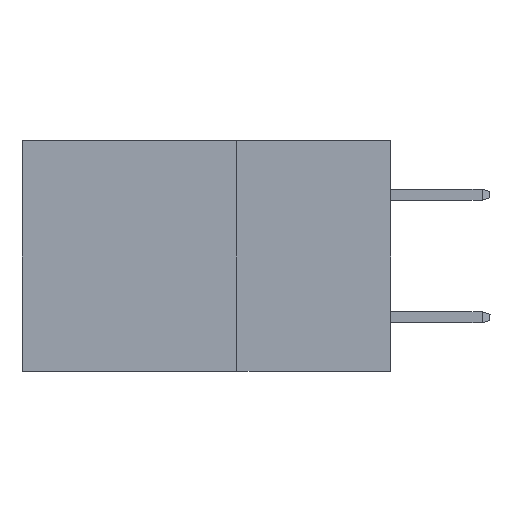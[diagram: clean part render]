
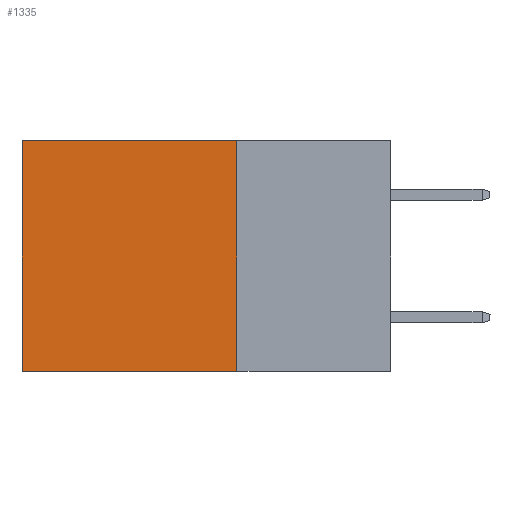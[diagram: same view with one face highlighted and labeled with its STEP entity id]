
A CAD part, left-side view. The second image highlights one B-rep face of the part: STEP entity #1335.
In plain terms, the highlighted planar face has unit normal (-1, 0, 0).
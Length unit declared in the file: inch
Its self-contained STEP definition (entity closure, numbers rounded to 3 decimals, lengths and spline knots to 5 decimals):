
#617 = FACE_OUTER_BOUND ( 'NONE', #4697, .T. ) ;
#1335 = ADVANCED_FACE ( 'NONE', ( #617 ), #15042, .F. ) ;
#1617 = DIRECTION ( 'NONE',  ( 0., 0., -1. ) ) ;
#1668 = DIRECTION ( 'NONE',  ( 0., 1., 0. ) ) ;
#1907 = CARTESIAN_POINT ( 'NONE',  ( 0.2875, 0.25, -0.375 ) ) ;
#2137 = LINE ( 'NONE', #16046, #6832 ) ;
#2836 = EDGE_CURVE ( 'NONE', #5734, #14524, #2137, .T. ) ;
#2960 = ORIENTED_EDGE ( 'NONE', *, *, #19787, .F. ) ;
#3759 = ORIENTED_EDGE ( 'NONE', *, *, #15949, .T. ) ;
#4549 = LINE ( 'NONE', #1907, #5886 ) ;
#4697 = EDGE_LOOP ( 'NONE', ( #3759, #7696, #2960, #5050 ) ) ;
#5050 = ORIENTED_EDGE ( 'NONE', *, *, #2836, .T. ) ;
#5734 = VERTEX_POINT ( 'NONE', #6624 ) ;
#5886 = VECTOR ( 'NONE', #1617, 39.37008 ) ;
#6001 = AXIS2_PLACEMENT_3D ( 'NONE', #15118, #16577, #8248 ) ;
#6624 = CARTESIAN_POINT ( 'NONE',  ( 0.2875, 0.25, 0. ) ) ;
#6832 = VECTOR ( 'NONE', #7786, 39.37008 ) ;
#7696 = ORIENTED_EDGE ( 'NONE', *, *, #13627, .F. ) ;
#7786 = DIRECTION ( 'NONE',  ( 0., 1., 0. ) ) ;
#8248 = DIRECTION ( 'NONE',  ( 0., 0., -1. ) ) ;
#9211 = DIRECTION ( 'NONE',  ( 0., 0., -1. ) ) ;
#11512 = VECTOR ( 'NONE', #1668, 39.37008 ) ;
#11729 = CARTESIAN_POINT ( 'NONE',  ( 0.2875, 0.25, -0.375 ) ) ;
#12411 = VERTEX_POINT ( 'NONE', #17726 ) ;
#13627 = EDGE_CURVE ( 'NONE', #12411, #15645, #17916, .T. ) ;
#14524 = VERTEX_POINT ( 'NONE', #17903 ) ;
#15042 = PLANE ( 'NONE',  #6001 ) ;
#15118 = CARTESIAN_POINT ( 'NONE',  ( 0.2875, 0.25, -0.375 ) ) ;
#15645 = VERTEX_POINT ( 'NONE', #17768 ) ;
#15949 = EDGE_CURVE ( 'NONE', #14524, #15645, #18079, .T. ) ;
#16046 = CARTESIAN_POINT ( 'NONE',  ( 0.2875, 0.25, 0. ) ) ;
#16468 = VECTOR ( 'NONE', #9211, 39.37008 ) ;
#16577 = DIRECTION ( 'NONE',  ( 1., 0., 0. ) ) ;
#17726 = CARTESIAN_POINT ( 'NONE',  ( 0.2875, 0.25, -0.375 ) ) ;
#17768 = CARTESIAN_POINT ( 'NONE',  ( 0.2875, 0.6, -0.375 ) ) ;
#17903 = CARTESIAN_POINT ( 'NONE',  ( 0.2875, 0.6, 0. ) ) ;
#17916 = LINE ( 'NONE', #11729, #11512 ) ;
#18079 = LINE ( 'NONE', #21298, #16468 ) ;
#19787 = EDGE_CURVE ( 'NONE', #5734, #12411, #4549, .T. ) ;
#21298 = CARTESIAN_POINT ( 'NONE',  ( 0.2875, 0.6, -0.375 ) ) ;
